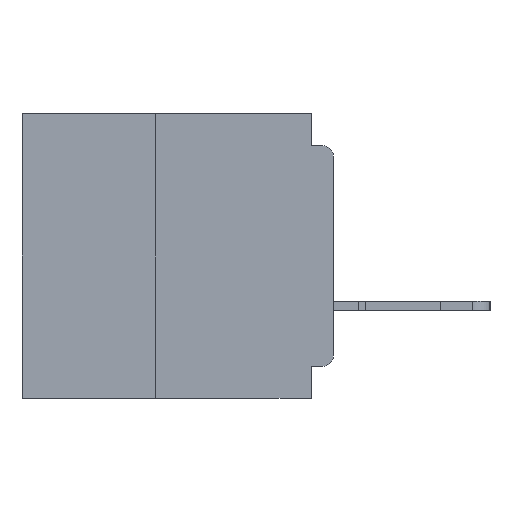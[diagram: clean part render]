
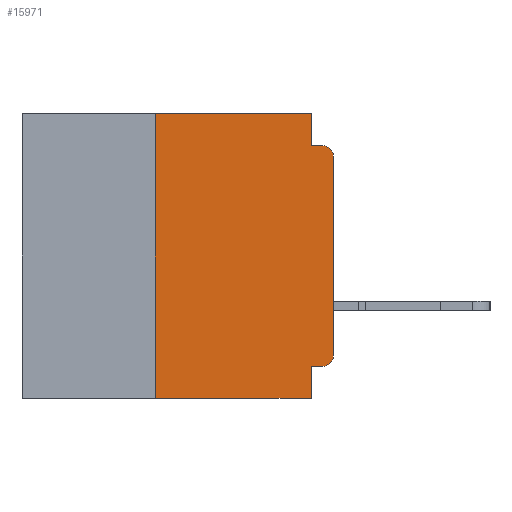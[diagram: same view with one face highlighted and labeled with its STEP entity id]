
A CAD part, left-side view. The second image highlights one B-rep face of the part: STEP entity #15971.
In plain terms, the highlighted planar face has unit normal (-1, 0, 0).
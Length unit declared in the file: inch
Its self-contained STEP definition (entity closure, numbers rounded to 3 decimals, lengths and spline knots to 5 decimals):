
#43 = DIRECTION ( 'NONE',  ( 0., -1., 0. ) ) ;
#1647 = VECTOR ( 'NONE', #41984, 39.37008 ) ;
#1732 = ORIENTED_EDGE ( 'NONE', *, *, #36865, .T. ) ;
#2135 = DIRECTION ( 'NONE',  ( 1., 0., 0. ) ) ;
#2203 = VERTEX_POINT ( 'NONE', #45463 ) ;
#2451 = VERTEX_POINT ( 'NONE', #27917 ) ;
#2782 = CARTESIAN_POINT ( 'NONE',  ( 0., 0.031, -0.045 ) ) ;
#3503 = DIRECTION ( 'NONE',  ( -1., 0., 0. ) ) ;
#3691 = EDGE_CURVE ( 'NONE', #33980, #41274, #47382, .T. ) ;
#4025 = CARTESIAN_POINT ( 'NONE',  ( 0., 0., -0.355 ) ) ;
#5474 = CARTESIAN_POINT ( 'NONE',  ( 0., 0., 0. ) ) ;
#5691 = VERTEX_POINT ( 'NONE', #7395 ) ;
#5887 = DIRECTION ( 'NONE',  ( -1., 0., 0. ) ) ;
#7180 = CARTESIAN_POINT ( 'NONE',  ( 0., 0.031, -0.4 ) ) ;
#7395 = CARTESIAN_POINT ( 'NONE',  ( 0., 0.25, 0. ) ) ;
#8415 = ORIENTED_EDGE ( 'NONE', *, *, #58337, .T. ) ;
#8991 = ORIENTED_EDGE ( 'NONE', *, *, #3691, .F. ) ;
#9596 = CARTESIAN_POINT ( 'NONE',  ( 0., 0.437, -0.4 ) ) ;
#10090 = ORIENTED_EDGE ( 'NONE', *, *, #12408, .T. ) ;
#10321 = DIRECTION ( 'NONE',  ( 0., 0., -1. ) ) ;
#10576 = VERTEX_POINT ( 'NONE', #14884 ) ;
#11533 = CARTESIAN_POINT ( 'NONE',  ( 0., 0.437, 0. ) ) ;
#12408 = EDGE_CURVE ( 'NONE', #25720, #2451, #56682, .T. ) ;
#12409 = EDGE_LOOP ( 'NONE', ( #10090, #1732, #8991, #48449, #55732, #19350, #40615, #41032, #52180, #8415 ) ) ;
#12531 = FACE_OUTER_BOUND ( 'NONE', #12409, .T. ) ;
#12899 = VECTOR ( 'NONE', #10321, 39.37008 ) ;
#13851 = VERTEX_POINT ( 'NONE', #39892 ) ;
#14579 = VECTOR ( 'NONE', #36273, 39.37008 ) ;
#14884 = CARTESIAN_POINT ( 'NONE',  ( 0., 0.015, -0.355 ) ) ;
#15971 = ADVANCED_FACE ( 'NONE', ( #12531 ), #21112, .F. ) ;
#17374 = CARTESIAN_POINT ( 'NONE',  ( 0., 0., -0.34 ) ) ;
#18025 = CARTESIAN_POINT ( 'NONE',  ( 0., 0.015, -0.045 ) ) ;
#19350 = ORIENTED_EDGE ( 'NONE', *, *, #25145, .F. ) ;
#19446 = EDGE_CURVE ( 'NONE', #26509, #33980, #25528, .T. ) ;
#20030 = CIRCLE ( 'NONE', #51378, 0.015 ) ;
#21112 = PLANE ( 'NONE',  #42690 ) ;
#21971 = CARTESIAN_POINT ( 'NONE',  ( 0., 0.25, -0.4 ) ) ;
#25145 = EDGE_CURVE ( 'NONE', #13851, #5691, #27210, .T. ) ;
#25452 = CIRCLE ( 'NONE', #54147, 0.015 ) ;
#25528 = LINE ( 'NONE', #29486, #12899 ) ;
#25720 = VERTEX_POINT ( 'NONE', #17374 ) ;
#25739 = VECTOR ( 'NONE', #43, 39.37008 ) ;
#26509 = VERTEX_POINT ( 'NONE', #42262 ) ;
#26988 = LINE ( 'NONE', #4025, #1647 ) ;
#27210 = LINE ( 'NONE', #21971, #14579 ) ;
#27917 = CARTESIAN_POINT ( 'NONE',  ( 0., 0., -0.06 ) ) ;
#28742 = LINE ( 'NONE', #9596, #25739 ) ;
#29411 = DIRECTION ( 'NONE',  ( 0., -1., 0. ) ) ;
#29486 = CARTESIAN_POINT ( 'NONE',  ( 0., 0.031, 0. ) ) ;
#29893 = CARTESIAN_POINT ( 'NONE',  ( 0., 0., -0.045 ) ) ;
#30623 = CARTESIAN_POINT ( 'NONE',  ( 0., 0.031, -0.4 ) ) ;
#31622 = VECTOR ( 'NONE', #57464, 39.37008 ) ;
#32040 = CARTESIAN_POINT ( 'NONE',  ( 0., 0.015, -0.06 ) ) ;
#32738 = VERTEX_POINT ( 'NONE', #30623 ) ;
#33980 = VERTEX_POINT ( 'NONE', #2782 ) ;
#34154 = EDGE_CURVE ( 'NONE', #10576, #2203, #26988, .T. ) ;
#34366 = CARTESIAN_POINT ( 'NONE',  ( 0., 0.015, -0.34 ) ) ;
#34871 = VECTOR ( 'NONE', #29411, 39.37008 ) ;
#35426 = DIRECTION ( 'NONE',  ( 0., 0., -1. ) ) ;
#36273 = DIRECTION ( 'NONE',  ( 0., 0., 1. ) ) ;
#36617 = DIRECTION ( 'NONE',  ( 0., -1., 0. ) ) ;
#36767 = DIRECTION ( 'NONE',  ( 0., 0., -1. ) ) ;
#36865 = EDGE_CURVE ( 'NONE', #2451, #41274, #20030, .T. ) ;
#39063 = DIRECTION ( 'NONE',  ( 0., 0., -1. ) ) ;
#39892 = CARTESIAN_POINT ( 'NONE',  ( 0., 0.25, -0.4 ) ) ;
#40615 = ORIENTED_EDGE ( 'NONE', *, *, #56173, .T. ) ;
#41032 = ORIENTED_EDGE ( 'NONE', *, *, #42863, .F. ) ;
#41274 = VERTEX_POINT ( 'NONE', #18025 ) ;
#41984 = DIRECTION ( 'NONE',  ( 0., 1., 0. ) ) ;
#42262 = CARTESIAN_POINT ( 'NONE',  ( 0., 0.031, 0. ) ) ;
#42690 = AXIS2_PLACEMENT_3D ( 'NONE', #11533, #2135, #35426 ) ;
#42863 = EDGE_CURVE ( 'NONE', #2203, #32738, #59020, .T. ) ;
#45463 = CARTESIAN_POINT ( 'NONE',  ( 0., 0.031, -0.355 ) ) ;
#46487 = VECTOR ( 'NONE', #49866, 39.37008 ) ;
#47382 = LINE ( 'NONE', #29893, #34871 ) ;
#48449 = ORIENTED_EDGE ( 'NONE', *, *, #19446, .F. ) ;
#48951 = LINE ( 'NONE', #60089, #59997 ) ;
#49866 = DIRECTION ( 'NONE',  ( 0., 0., -1. ) ) ;
#51378 = AXIS2_PLACEMENT_3D ( 'NONE', #32040, #3503, #36767 ) ;
#52180 = ORIENTED_EDGE ( 'NONE', *, *, #34154, .F. ) ;
#54147 = AXIS2_PLACEMENT_3D ( 'NONE', #34366, #5887, #39063 ) ;
#54519 = EDGE_CURVE ( 'NONE', #5691, #26509, #48951, .T. ) ;
#55732 = ORIENTED_EDGE ( 'NONE', *, *, #54519, .F. ) ;
#56173 = EDGE_CURVE ( 'NONE', #13851, #32738, #28742, .T. ) ;
#56682 = LINE ( 'NONE', #5474, #31622 ) ;
#57464 = DIRECTION ( 'NONE',  ( 0., 0., 1. ) ) ;
#58337 = EDGE_CURVE ( 'NONE', #10576, #25720, #25452, .T. ) ;
#59020 = LINE ( 'NONE', #7180, #46487 ) ;
#59997 = VECTOR ( 'NONE', #36617, 39.37008 ) ;
#60089 = CARTESIAN_POINT ( 'NONE',  ( 0., 0.437, 0. ) ) ;
